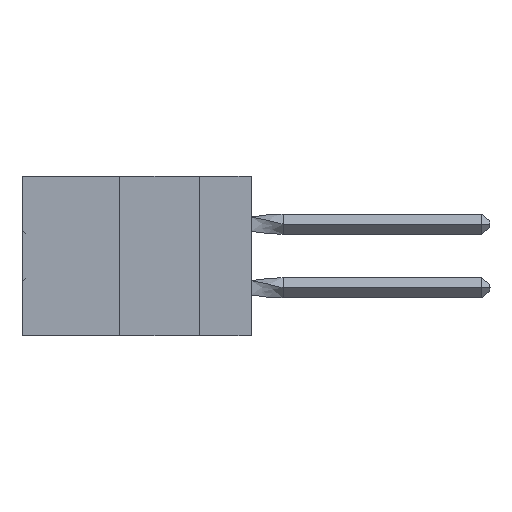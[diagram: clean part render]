
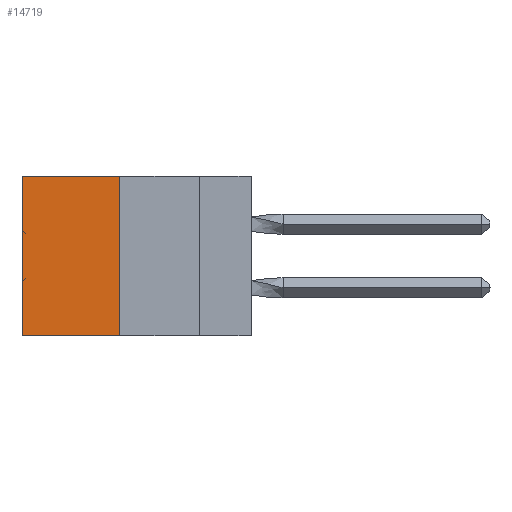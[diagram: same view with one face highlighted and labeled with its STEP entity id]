
A CAD part, left-side view. The second image highlights one B-rep face of the part: STEP entity #14719.
In plain terms, the highlighted planar face has unit normal (-1, 0, 0).
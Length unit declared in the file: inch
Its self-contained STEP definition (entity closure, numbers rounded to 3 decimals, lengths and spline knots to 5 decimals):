
#892 = CARTESIAN_POINT ( 'NONE',  ( 0.305, 0.72, 0. ) ) ;
#3513 = ORIENTED_EDGE ( 'NONE', *, *, #32052, .T. ) ;
#3851 = DIRECTION ( 'NONE',  ( 0., 1., 0. ) ) ;
#3913 = VERTEX_POINT ( 'NONE', #41298 ) ;
#8044 = VERTEX_POINT ( 'NONE', #892 ) ;
#9071 = DIRECTION ( 'NONE',  ( 1., 0., 0. ) ) ;
#14581 = VECTOR ( 'NONE', #35754, 39.37008 ) ;
#14719 = ADVANCED_FACE ( 'NONE', ( #44653 ), #53818, .F. ) ;
#15111 = VERTEX_POINT ( 'NONE', #35288 ) ;
#15244 = VECTOR ( 'NONE', #3851, 39.37008 ) ;
#15307 = CARTESIAN_POINT ( 'NONE',  ( 0.305, 0.413, -0.5 ) ) ;
#16389 = VECTOR ( 'NONE', #30199, 39.37008 ) ;
#16614 = AXIS2_PLACEMENT_3D ( 'NONE', #51264, #9071, #53221 ) ;
#20523 = VERTEX_POINT ( 'NONE', #21147 ) ;
#20953 = CARTESIAN_POINT ( 'NONE',  ( 0.305, 0.72, -0.5 ) ) ;
#21147 = CARTESIAN_POINT ( 'NONE',  ( 0.305, 0.413, 0. ) ) ;
#30199 = DIRECTION ( 'NONE',  ( 0., 0., -1. ) ) ;
#31448 = CARTESIAN_POINT ( 'NONE',  ( 0.305, 0.413, -0.5 ) ) ;
#32052 = EDGE_CURVE ( 'NONE', #8044, #15111, #47952, .T. ) ;
#33068 = EDGE_CURVE ( 'NONE', #20523, #3913, #47562, .T. ) ;
#34018 = ORIENTED_EDGE ( 'NONE', *, *, #33068, .F. ) ;
#35288 = CARTESIAN_POINT ( 'NONE',  ( 0.305, 0.72, -0.5 ) ) ;
#35754 = DIRECTION ( 'NONE',  ( 0., 0., -1. ) ) ;
#37117 = VECTOR ( 'NONE', #50782, 39.37008 ) ;
#41298 = CARTESIAN_POINT ( 'NONE',  ( 0.305, 0.413, -0.5 ) ) ;
#42352 = EDGE_CURVE ( 'NONE', #3913, #15111, #48316, .T. ) ;
#43428 = ORIENTED_EDGE ( 'NONE', *, *, #42352, .F. ) ;
#44653 = FACE_OUTER_BOUND ( 'NONE', #45655, .T. ) ;
#45655 = EDGE_LOOP ( 'NONE', ( #3513, #43428, #34018, #53180 ) ) ;
#47562 = LINE ( 'NONE', #31448, #14581 ) ;
#47952 = LINE ( 'NONE', #20953, #16389 ) ;
#48316 = LINE ( 'NONE', #15307, #37117 ) ;
#50782 = DIRECTION ( 'NONE',  ( 0., 1., 0. ) ) ;
#51264 = CARTESIAN_POINT ( 'NONE',  ( 0.305, 0.413, -0.5 ) ) ;
#53180 = ORIENTED_EDGE ( 'NONE', *, *, #54422, .T. ) ;
#53221 = DIRECTION ( 'NONE',  ( 0., 0., -1. ) ) ;
#53818 = PLANE ( 'NONE',  #16614 ) ;
#53841 = CARTESIAN_POINT ( 'NONE',  ( 0.305, 0.413, 0. ) ) ;
#54422 = EDGE_CURVE ( 'NONE', #20523, #8044, #55922, .T. ) ;
#55922 = LINE ( 'NONE', #53841, #15244 ) ;
